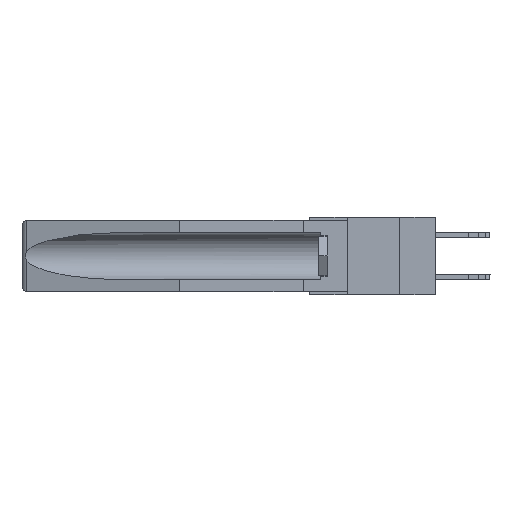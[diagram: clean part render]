
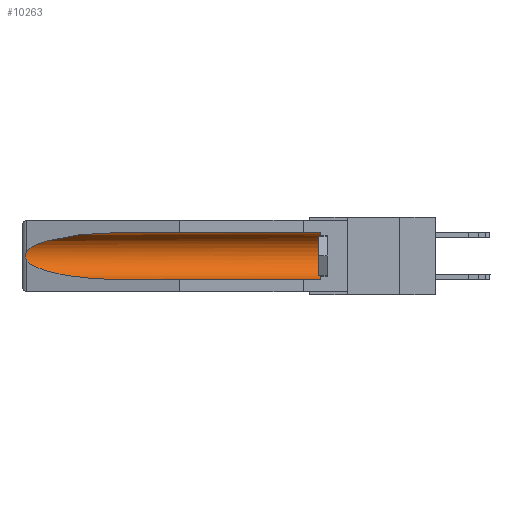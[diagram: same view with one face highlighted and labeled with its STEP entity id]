
A CAD part, left-side view. The second image highlights one B-rep face of the part: STEP entity #10263.
In plain terms, the highlighted cylindrical face has radius 2.857 mm (diameter 5.715 mm), a partial arc.
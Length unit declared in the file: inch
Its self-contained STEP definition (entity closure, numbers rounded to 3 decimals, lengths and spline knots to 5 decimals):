
#110 =( BOUNDED_CURVE ( )  B_SPLINE_CURVE ( 3, ( #4951, #16506, #11666, #16211 ),
 .UNSPECIFIED., .F., .F. ) 
 B_SPLINE_CURVE_WITH_KNOTS ( ( 4, 4 ),
 ( 0.1948, 1.5708 ),
 .UNSPECIFIED. ) 
 CURVE ( )  GEOMETRIC_REPRESENTATION_ITEM ( )  RATIONAL_B_SPLINE_CURVE ( ( 1., 0.848, 0.848, 1. ) ) 
 REPRESENTATION_ITEM ( '' )  );
#389 = EDGE_CURVE ( 'NONE', #12510, #9771, #14872, .T. ) ;
#739 = CIRCLE ( 'NONE', #15382, 0.1125 ) ;
#1689 = CARTESIAN_POINT ( 'NONE',  ( 0.155, 0.126, -0.059 ) ) ;
#1940 = CARTESIAN_POINT ( 'NONE',  ( 0.26537, 1.52718, -0.14972 ) ) ;
#2020 = CYLINDRICAL_SURFACE ( 'NONE', #14328, 0.1125 ) ;
#2292 = CARTESIAN_POINT ( 'NONE',  ( 0.26655, 1.53094, -0.18657 ) ) ;
#2410 = CARTESIAN_POINT ( 'NONE',  ( 0.26537, 1.52718, -0.14972 ) ) ;
#2431 = CARTESIAN_POINT ( 'NONE',  ( 0.155, -0.30754, -0.284 ) ) ;
#2464 = VECTOR ( 'NONE', #8694, 39.37008 ) ;
#2727 = EDGE_CURVE ( 'NONE', #6147, #19351, #110, .T. ) ;
#2859 = CARTESIAN_POINT ( 'NONE',  ( 0.26537, 1.52718, -0.19328 ) ) ;
#2880 = ORIENTED_EDGE ( 'NONE', *, *, #15557, .T. ) ;
#3409 = CARTESIAN_POINT ( 'NONE',  ( 0.155, -0.30754, -0.1715 ) ) ;
#3963 = CARTESIAN_POINT ( 'NONE',  ( 0.155, 1.07973, -0.059 ) ) ;
#4951 = CARTESIAN_POINT ( 'NONE',  ( 0.26537, 1.52718, -0.19328 ) ) ;
#4976 = DIRECTION ( 'NONE',  ( 0., 0., 1. ) ) ;
#5412 = CARTESIAN_POINT ( 'NONE',  ( 0.2673, 1.5327, -0.16383 ) ) ;
#5854 = EDGE_CURVE ( 'NONE', #16512, #17127, #739, .T. ) ;
#6147 = VERTEX_POINT ( 'NONE', #2859 ) ;
#6589 = ORIENTED_EDGE ( 'NONE', *, *, #16129, .F. ) ;
#7006 = ORIENTED_EDGE ( 'NONE', *, *, #2727, .T. ) ;
#7080 = CARTESIAN_POINT ( 'NONE',  ( 0.2673, 1.53269, -0.17917 ) ) ;
#7181 = CARTESIAN_POINT ( 'NONE',  ( 0.25451, 1.48313, -0.09465 ) ) ;
#7213 = CARTESIAN_POINT ( 'NONE',  ( 0.26597, 1.52961, -0.15275 ) ) ;
#7255 = EDGE_LOOP ( 'NONE', ( #13915, #15110, #7006, #6589, #9086, #2880 ) ) ;
#7751 = CARTESIAN_POINT ( 'NONE',  ( 0.155, 0.126, -0.284 ) ) ;
#7880 = DIRECTION ( 'NONE',  ( 0., -1., 0. ) ) ;
#8549 = CARTESIAN_POINT ( 'NONE',  ( 0.2675, 1.53308, -0.17534 ) ) ;
#8694 = DIRECTION ( 'NONE',  ( 0., 1., 0. ) ) ;
#9086 = ORIENTED_EDGE ( 'NONE', *, *, #5854, .T. ) ;
#9121 = CARTESIAN_POINT ( 'NONE',  ( 0.155, 1.07973, -0.059 ) ) ;
#9771 = VERTEX_POINT ( 'NONE', #1940 ) ;
#10222 = VECTOR ( 'NONE', #16400, 39.37008 ) ;
#10263 = ADVANCED_FACE ( 'NONE', ( #18158 ), #2020, .F. ) ;
#11666 = CARTESIAN_POINT ( 'NONE',  ( 0.21114, 1.30732, -0.284 ) ) ;
#11934 = CARTESIAN_POINT ( 'NONE',  ( 0.155, -0.30754, -0.059 ) ) ;
#12510 = VERTEX_POINT ( 'NONE', #9121 ) ;
#12851 = CARTESIAN_POINT ( 'NONE',  ( 0.155, 0.126, -0.1715 ) ) ;
#13915 = ORIENTED_EDGE ( 'NONE', *, *, #389, .T. ) ;
#14328 = AXIS2_PLACEMENT_3D ( 'NONE', #3409, #14576, #4976 ) ;
#14576 = DIRECTION ( 'NONE',  ( 0., 1., 0. ) ) ;
#14591 = B_SPLINE_CURVE_WITH_KNOTS ( 'NONE', 3,
 ( #18345, #7213, #16625, #5412, #16755, #8549, #7080, #2292, #19810, #18419 ),
 .UNSPECIFIED., .F., .F.,
 ( 4, 2, 2, 2, 4 ),
 ( 0., 0.00029, 0.00058, 0.00087, 0.00117 ),
 .UNSPECIFIED. ) ;
#14872 =( BOUNDED_CURVE ( )  B_SPLINE_CURVE ( 3, ( #3963, #16867, #7181, #2410 ),
 .UNSPECIFIED., .F., .F. ) 
 B_SPLINE_CURVE_WITH_KNOTS ( ( 4, 4 ),
 ( 4.71239, 6.08839 ),
 .UNSPECIFIED. ) 
 CURVE ( )  GEOMETRIC_REPRESENTATION_ITEM ( )  RATIONAL_B_SPLINE_CURVE ( ( 1., 0.848, 0.848, 1. ) ) 
 REPRESENTATION_ITEM ( '' )  );
#15110 = ORIENTED_EDGE ( 'NONE', *, *, #17965, .T. ) ;
#15382 = AXIS2_PLACEMENT_3D ( 'NONE', #12851, #7880, #19357 ) ;
#15557 = EDGE_CURVE ( 'NONE', #17127, #12510, #16333, .T. ) ;
#16129 = EDGE_CURVE ( 'NONE', #16512, #19351, #17542, .T. ) ;
#16211 = CARTESIAN_POINT ( 'NONE',  ( 0.155, 1.07973, -0.284 ) ) ;
#16333 = LINE ( 'NONE', #11934, #2464 ) ;
#16400 = DIRECTION ( 'NONE',  ( 0., 1., 0. ) ) ;
#16506 = CARTESIAN_POINT ( 'NONE',  ( 0.25451, 1.48313, -0.24835 ) ) ;
#16512 = VERTEX_POINT ( 'NONE', #7751 ) ;
#16625 = CARTESIAN_POINT ( 'NONE',  ( 0.26654, 1.53092, -0.15636 ) ) ;
#16755 = CARTESIAN_POINT ( 'NONE',  ( 0.2675, 1.53308, -0.16763 ) ) ;
#16867 = CARTESIAN_POINT ( 'NONE',  ( 0.21114, 1.30732, -0.059 ) ) ;
#17127 = VERTEX_POINT ( 'NONE', #1689 ) ;
#17542 = LINE ( 'NONE', #2431, #10222 ) ;
#17922 = CARTESIAN_POINT ( 'NONE',  ( 0.155, 1.07973, -0.284 ) ) ;
#17965 = EDGE_CURVE ( 'NONE', #9771, #6147, #14591, .T. ) ;
#18158 = FACE_OUTER_BOUND ( 'NONE', #7255, .T. ) ;
#18345 = CARTESIAN_POINT ( 'NONE',  ( 0.26537, 1.52718, -0.14972 ) ) ;
#18419 = CARTESIAN_POINT ( 'NONE',  ( 0.26537, 1.52718, -0.19328 ) ) ;
#19351 = VERTEX_POINT ( 'NONE', #17922 ) ;
#19357 = DIRECTION ( 'NONE',  ( 0., 0., 1. ) ) ;
#19810 = CARTESIAN_POINT ( 'NONE',  ( 0.26597, 1.5296, -0.19026 ) ) ;
